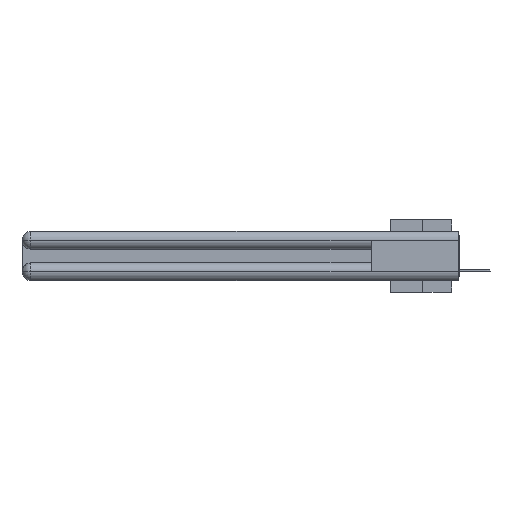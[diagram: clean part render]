
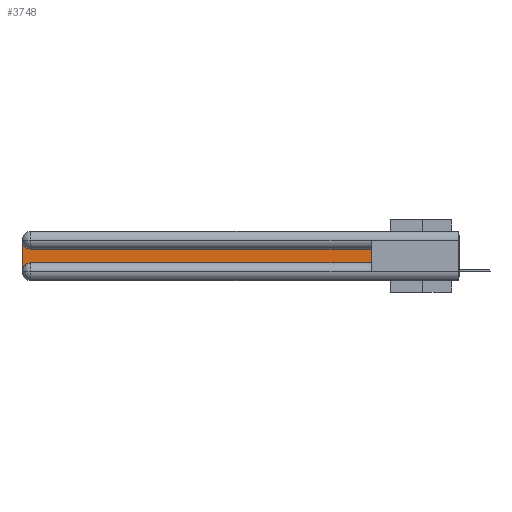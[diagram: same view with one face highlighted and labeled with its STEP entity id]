
A CAD part, left-side view. The second image highlights one B-rep face of the part: STEP entity #3748.
In plain terms, the highlighted planar face has unit normal (-1, 0, 0).
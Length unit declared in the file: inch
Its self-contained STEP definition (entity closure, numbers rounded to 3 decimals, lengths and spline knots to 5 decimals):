
#201 = EDGE_CURVE ( 'NONE', #27161, #19860, #17180, .T. ) ;
#1408 = CARTESIAN_POINT ( 'NONE',  ( 0.075, 0.6, -0.2175 ) ) ;
#1832 = ORIENTED_EDGE ( 'NONE', *, *, #6534, .T. ) ;
#3748 = ADVANCED_FACE ( 'NONE', ( #30374 ), #15363, .F. ) ;
#4985 = VERTEX_POINT ( 'NONE', #13800 ) ;
#6534 = EDGE_CURVE ( 'NONE', #11117, #4985, #27897, .T. ) ;
#6576 = ORIENTED_EDGE ( 'NONE', *, *, #9201, .T. ) ;
#9079 = CARTESIAN_POINT ( 'NONE',  ( 0.075, 0.6, -0.2175 ) ) ;
#9154 = DIRECTION ( 'NONE',  ( 1., 0., 0. ) ) ;
#9201 = EDGE_CURVE ( 'NONE', #19860, #11117, #15365, .T. ) ;
#9514 = DIRECTION ( 'NONE',  ( 1., 0., 0. ) ) ;
#10090 = LINE ( 'NONE', #9079, #22457 ) ;
#10228 = VECTOR ( 'NONE', #27172, 39.37008 ) ;
#10673 = ORIENTED_EDGE ( 'NONE', *, *, #11083, .T. ) ;
#11083 = EDGE_CURVE ( 'NONE', #16649, #11627, #12566, .T. ) ;
#11117 = VERTEX_POINT ( 'NONE', #29660 ) ;
#11481 = EDGE_LOOP ( 'NONE', ( #10673, #20132, #15052, #6576, #1832, #15617 ) ) ;
#11627 = VERTEX_POINT ( 'NONE', #30239 ) ;
#12195 = CARTESIAN_POINT ( 'NONE',  ( 0.075, 2.94, -0.2775 ) ) ;
#12566 = LINE ( 'NONE', #17251, #10228 ) ;
#13776 = DIRECTION ( 'NONE',  ( 0., -1., 0. ) ) ;
#13800 = CARTESIAN_POINT ( 'NONE',  ( 0.075, 0.6, -0.2175 ) ) ;
#14540 = DIRECTION ( 'NONE',  ( 0., 0., -1. ) ) ;
#15052 = ORIENTED_EDGE ( 'NONE', *, *, #201, .T. ) ;
#15184 = DIRECTION ( 'NONE',  ( 0., 0., -1. ) ) ;
#15363 = PLANE ( 'NONE',  #24714 ) ;
#15365 = CIRCLE ( 'NONE', #28565, 0.06 ) ;
#15617 = ORIENTED_EDGE ( 'NONE', *, *, #26615, .T. ) ;
#16629 = DIRECTION ( 'NONE',  ( 0., 0., 1. ) ) ;
#16649 = VERTEX_POINT ( 'NONE', #29625 ) ;
#16952 = DIRECTION ( 'NONE',  ( 0., 0., -1. ) ) ;
#17128 = CIRCLE ( 'NONE', #17777, 0.06 ) ;
#17162 = CARTESIAN_POINT ( 'NONE',  ( 0.075, 3., -0.1225 ) ) ;
#17180 = LINE ( 'NONE', #22098, #22200 ) ;
#17251 = CARTESIAN_POINT ( 'NONE',  ( 0.075, 0.6, -0.1225 ) ) ;
#17777 = AXIS2_PLACEMENT_3D ( 'NONE', #26616, #9154, #29209 ) ;
#19860 = VERTEX_POINT ( 'NONE', #29886 ) ;
#20132 = ORIENTED_EDGE ( 'NONE', *, *, #25370, .T. ) ;
#22098 = CARTESIAN_POINT ( 'NONE',  ( 0.075, 3., -0.2175 ) ) ;
#22200 = VECTOR ( 'NONE', #15184, 39.37008 ) ;
#22457 = VECTOR ( 'NONE', #16629, 39.37008 ) ;
#24714 = AXIS2_PLACEMENT_3D ( 'NONE', #17162, #9514, #16952 ) ;
#25370 = EDGE_CURVE ( 'NONE', #11627, #27161, #17128, .T. ) ;
#26209 = CARTESIAN_POINT ( 'NONE',  ( 0.075, 3., -0.0625 ) ) ;
#26615 = EDGE_CURVE ( 'NONE', #4985, #16649, #10090, .T. ) ;
#26616 = CARTESIAN_POINT ( 'NONE',  ( 0.075, 2.94, -0.0625 ) ) ;
#27161 = VERTEX_POINT ( 'NONE', #26209 ) ;
#27172 = DIRECTION ( 'NONE',  ( 0., 1., 0. ) ) ;
#27897 = LINE ( 'NONE', #1408, #30622 ) ;
#28565 = AXIS2_PLACEMENT_3D ( 'NONE', #12195, #29230, #14540 ) ;
#29209 = DIRECTION ( 'NONE',  ( 0., 0., -1. ) ) ;
#29230 = DIRECTION ( 'NONE',  ( 1., 0., 0. ) ) ;
#29625 = CARTESIAN_POINT ( 'NONE',  ( 0.075, 0.6, -0.1225 ) ) ;
#29660 = CARTESIAN_POINT ( 'NONE',  ( 0.075, 2.94, -0.2175 ) ) ;
#29886 = CARTESIAN_POINT ( 'NONE',  ( 0.075, 3., -0.2775 ) ) ;
#30239 = CARTESIAN_POINT ( 'NONE',  ( 0.075, 2.94, -0.1225 ) ) ;
#30374 = FACE_OUTER_BOUND ( 'NONE', #11481, .T. ) ;
#30622 = VECTOR ( 'NONE', #13776, 39.37008 ) ;
